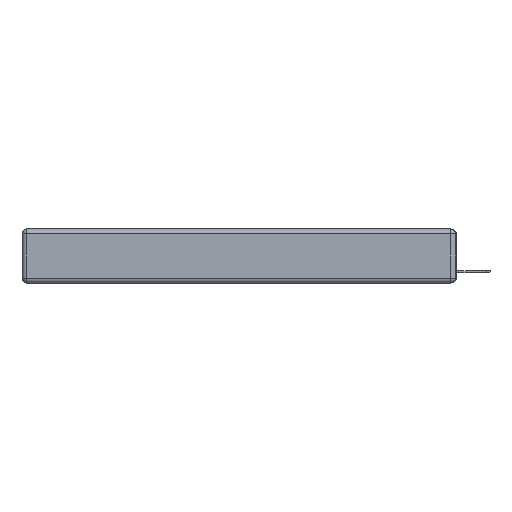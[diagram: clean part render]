
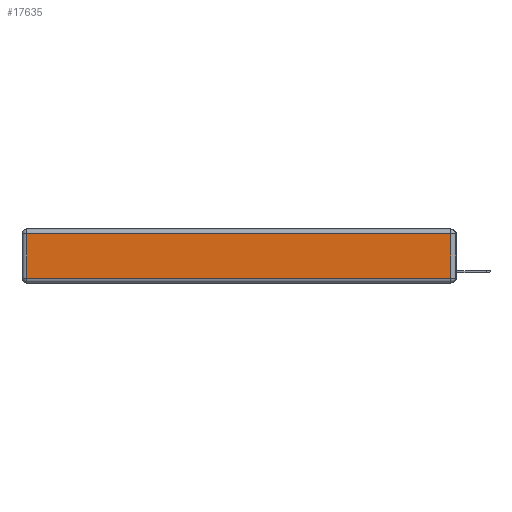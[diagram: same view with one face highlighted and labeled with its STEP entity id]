
A CAD part, left-side view. The second image highlights one B-rep face of the part: STEP entity #17635.
In plain terms, the highlighted planar face has unit normal (-1, 0, 0).
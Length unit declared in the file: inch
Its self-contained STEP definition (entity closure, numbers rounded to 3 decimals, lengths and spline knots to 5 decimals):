
#94 = CARTESIAN_POINT ( 'NONE',  ( 0., 2.72, -0.03 ) ) ;
#188 = DIRECTION ( 'NONE',  ( 0., -1., 0. ) ) ;
#428 = VECTOR ( 'NONE', #10354, 39.37008 ) ;
#3135 = LINE ( 'NONE', #10105, #3361 ) ;
#3137 = ORIENTED_EDGE ( 'NONE', *, *, #4968, .T. ) ;
#3361 = VECTOR ( 'NONE', #21410, 39.37008 ) ;
#3504 = CARTESIAN_POINT ( 'NONE',  ( 0., 0., -0.313 ) ) ;
#3645 = CARTESIAN_POINT ( 'NONE',  ( 0., 0., -0.343 ) ) ;
#4580 = CARTESIAN_POINT ( 'NONE',  ( 0., 2.72, -0.313 ) ) ;
#4968 = EDGE_CURVE ( 'NONE', #11539, #13833, #17786, .T. ) ;
#5362 = DIRECTION ( 'NONE',  ( 0., 0., 1. ) ) ;
#5877 = ORIENTED_EDGE ( 'NONE', *, *, #18182, .T. ) ;
#6331 = EDGE_LOOP ( 'NONE', ( #3137, #8092, #16942, #5877 ) ) ;
#7352 = EDGE_CURVE ( 'NONE', #17012, #17671, #16975, .T. ) ;
#8092 = ORIENTED_EDGE ( 'NONE', *, *, #22574, .T. ) ;
#8787 = DIRECTION ( 'NONE',  ( -1., 0., 0. ) ) ;
#8906 = PLANE ( 'NONE',  #14061 ) ;
#9281 = VECTOR ( 'NONE', #10312, 39.37008 ) ;
#10105 = CARTESIAN_POINT ( 'NONE',  ( 0., 0.03, -0.343 ) ) ;
#10312 = DIRECTION ( 'NONE',  ( 0., 0., -1. ) ) ;
#10354 = DIRECTION ( 'NONE',  ( 0., 1., 0. ) ) ;
#11539 = VERTEX_POINT ( 'NONE', #4580 ) ;
#13533 = CARTESIAN_POINT ( 'NONE',  ( 0., 0.03, -0.313 ) ) ;
#13833 = VERTEX_POINT ( 'NONE', #13533 ) ;
#14061 = AXIS2_PLACEMENT_3D ( 'NONE', #3645, #8787, #5362 ) ;
#15337 = CARTESIAN_POINT ( 'NONE',  ( 0., 2.72, -0.343 ) ) ;
#15685 = VECTOR ( 'NONE', #188, 39.37008 ) ;
#16942 = ORIENTED_EDGE ( 'NONE', *, *, #7352, .T. ) ;
#16975 = LINE ( 'NONE', #20649, #428 ) ;
#17012 = VERTEX_POINT ( 'NONE', #19925 ) ;
#17635 = ADVANCED_FACE ( 'NONE', ( #21681 ), #8906, .T. ) ;
#17671 = VERTEX_POINT ( 'NONE', #94 ) ;
#17786 = LINE ( 'NONE', #3504, #15685 ) ;
#18182 = EDGE_CURVE ( 'NONE', #17671, #11539, #18870, .T. ) ;
#18870 = LINE ( 'NONE', #15337, #9281 ) ;
#19925 = CARTESIAN_POINT ( 'NONE',  ( 0., 0.03, -0.03 ) ) ;
#20649 = CARTESIAN_POINT ( 'NONE',  ( 0., 2.75, -0.03 ) ) ;
#21410 = DIRECTION ( 'NONE',  ( 0., 0., 1. ) ) ;
#21681 = FACE_OUTER_BOUND ( 'NONE', #6331, .T. ) ;
#22574 = EDGE_CURVE ( 'NONE', #13833, #17012, #3135, .T. ) ;
